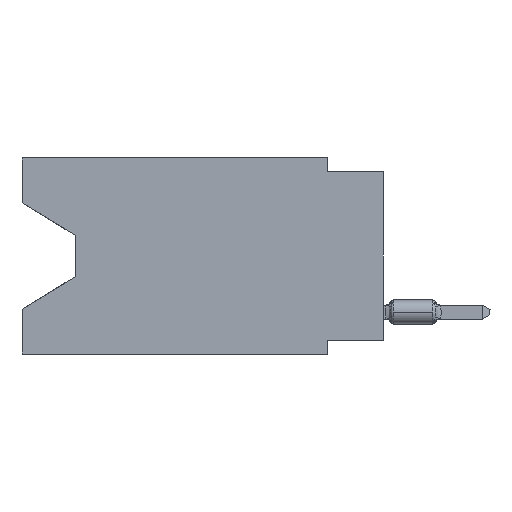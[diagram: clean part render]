
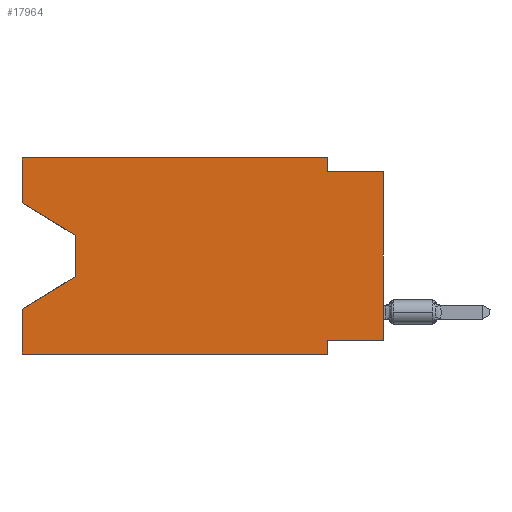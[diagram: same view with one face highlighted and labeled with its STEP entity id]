
A CAD part, left-side view. The second image highlights one B-rep face of the part: STEP entity #17964.
In plain terms, the highlighted planar face has unit normal (-1, 0, 0).
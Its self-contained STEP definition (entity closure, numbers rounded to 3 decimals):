
#676 = CARTESIAN_POINT ( 'NONE',  ( 0., 2.54, -0.635 ) ) ;
#875 = DIRECTION ( 'NONE',  ( 0., 0., -1. ) ) ;
#980 = VECTOR ( 'NONE', #48098, 1000. ) ;
#1937 = VECTOR ( 'NONE', #20062, 1000. ) ;
#3966 = VECTOR ( 'NONE', #53727, 1000. ) ;
#4499 = EDGE_CURVE ( 'NONE', #33399, #41861, #5363, .T. ) ;
#4623 = LINE ( 'NONE', #45652, #40477 ) ;
#4881 = CARTESIAN_POINT ( 'NONE',  ( 0., 2.54, -8.89 ) ) ;
#5284 = CARTESIAN_POINT ( 'NONE',  ( 0., 0., -8.255 ) ) ;
#5363 = LINE ( 'NONE', #25217, #5516 ) ;
#5516 = VECTOR ( 'NONE', #49638, 1000. ) ;
#5627 = AXIS2_PLACEMENT_3D ( 'NONE', #17727, #50053, #875 ) ;
#6495 = ORIENTED_EDGE ( 'NONE', *, *, #13735, .F. ) ;
#6809 = DIRECTION ( 'NONE',  ( 0., -1., 0. ) ) ;
#7273 = CARTESIAN_POINT ( 'NONE',  ( 0., 13.97, -5.385 ) ) ;
#8082 = LINE ( 'NONE', #28492, #21267 ) ;
#8533 = VERTEX_POINT ( 'NONE', #39669 ) ;
#8679 = LINE ( 'NONE', #4881, #52269 ) ;
#10050 = VERTEX_POINT ( 'NONE', #676 ) ;
#10669 = ORIENTED_EDGE ( 'NONE', *, *, #30252, .F. ) ;
#11470 = VECTOR ( 'NONE', #51185, 1000. ) ;
#11529 = VERTEX_POINT ( 'NONE', #7273 ) ;
#11612 = VERTEX_POINT ( 'NONE', #30562 ) ;
#12620 = VECTOR ( 'NONE', #21866, 1000. ) ;
#13368 = PLANE ( 'NONE',  #5627 ) ;
#13735 = EDGE_CURVE ( 'NONE', #29307, #45495, #52917, .T. ) ;
#14941 = LINE ( 'NONE', #31545, #980 ) ;
#15012 = LINE ( 'NONE', #20177, #34600 ) ;
#16884 = CARTESIAN_POINT ( 'NONE',  ( 0., 16.383, 0. ) ) ;
#17579 = ORIENTED_EDGE ( 'NONE', *, *, #43287, .T. ) ;
#17727 = CARTESIAN_POINT ( 'NONE',  ( 0., 16.383, 0. ) ) ;
#17964 = ADVANCED_FACE ( 'NONE', ( #42196 ), #13368, .F. ) ;
#18156 = VECTOR ( 'NONE', #37771, 1000. ) ;
#19597 = EDGE_CURVE ( 'NONE', #11529, #21033, #4623, .T. ) ;
#20062 = DIRECTION ( 'NONE',  ( 0., 0., 1. ) ) ;
#20177 = CARTESIAN_POINT ( 'NONE',  ( 0., 0., -0.635 ) ) ;
#20643 = LINE ( 'NONE', #25277, #18156 ) ;
#21033 = VERTEX_POINT ( 'NONE', #52001 ) ;
#21267 = VECTOR ( 'NONE', #45060, 1000. ) ;
#21480 = DIRECTION ( 'NONE',  ( 0., 0.855, -0.519 ) ) ;
#21866 = DIRECTION ( 'NONE',  ( 0., 0., 1. ) ) ;
#21906 = CARTESIAN_POINT ( 'NONE',  ( 0., 2.54, -8.89 ) ) ;
#24367 = CARTESIAN_POINT ( 'NONE',  ( 0., 13.97, -3.505 ) ) ;
#25217 = CARTESIAN_POINT ( 'NONE',  ( 0., 16.383, -8.89 ) ) ;
#25277 = CARTESIAN_POINT ( 'NONE',  ( 0., 2.54, 0. ) ) ;
#25775 = EDGE_CURVE ( 'NONE', #29307, #40229, #14941, .T. ) ;
#26586 = EDGE_CURVE ( 'NONE', #10050, #11612, #15012, .T. ) ;
#27057 = EDGE_CURVE ( 'NONE', #8533, #10050, #20643, .T. ) ;
#27648 = EDGE_CURVE ( 'NONE', #45495, #8533, #28547, .T. ) ;
#28492 = CARTESIAN_POINT ( 'NONE',  ( 0., 13.97, -3.505 ) ) ;
#28547 = LINE ( 'NONE', #48644, #28632 ) ;
#28632 = VECTOR ( 'NONE', #6809, 1000. ) ;
#29307 = VERTEX_POINT ( 'NONE', #49099 ) ;
#30143 = ORIENTED_EDGE ( 'NONE', *, *, #42589, .T. ) ;
#30252 = EDGE_CURVE ( 'NONE', #50317, #41861, #8679, .T. ) ;
#30560 = LINE ( 'NONE', #38455, #12620 ) ;
#30562 = CARTESIAN_POINT ( 'NONE',  ( 0., 0., -0.635 ) ) ;
#31545 = CARTESIAN_POINT ( 'NONE',  ( 0., 16.383, -2.038 ) ) ;
#33121 = ORIENTED_EDGE ( 'NONE', *, *, #50283, .F. ) ;
#33399 = VERTEX_POINT ( 'NONE', #51357 ) ;
#33839 = CARTESIAN_POINT ( 'NONE',  ( 0., 2.54, -8.255 ) ) ;
#34078 = ORIENTED_EDGE ( 'NONE', *, *, #27057, .F. ) ;
#34600 = VECTOR ( 'NONE', #36224, 1000. ) ;
#36135 = ORIENTED_EDGE ( 'NONE', *, *, #26586, .F. ) ;
#36224 = DIRECTION ( 'NONE',  ( 0., -1., 0. ) ) ;
#37077 = ORIENTED_EDGE ( 'NONE', *, *, #25775, .T. ) ;
#37194 = LINE ( 'NONE', #45340, #3966 ) ;
#37394 = VERTEX_POINT ( 'NONE', #42580 ) ;
#37771 = DIRECTION ( 'NONE',  ( 0., 0., -1. ) ) ;
#38455 = CARTESIAN_POINT ( 'NONE',  ( 0., 16.383, 0. ) ) ;
#38637 = ORIENTED_EDGE ( 'NONE', *, *, #27648, .F. ) ;
#38867 = DIRECTION ( 'NONE',  ( 0., 0., -1. ) ) ;
#39669 = CARTESIAN_POINT ( 'NONE',  ( 0., 2.54, 0. ) ) ;
#40229 = VERTEX_POINT ( 'NONE', #24367 ) ;
#40477 = VECTOR ( 'NONE', #21480, 1000. ) ;
#41279 = ORIENTED_EDGE ( 'NONE', *, *, #4499, .T. ) ;
#41861 = VERTEX_POINT ( 'NONE', #21906 ) ;
#42196 = FACE_OUTER_BOUND ( 'NONE', #42490, .T. ) ;
#42490 = EDGE_LOOP ( 'NONE', ( #37077, #17579, #51332, #33121, #41279, #10669, #43118, #30143, #36135, #34078, #38637, #6495 ) ) ;
#42580 = CARTESIAN_POINT ( 'NONE',  ( 0., 0., -8.255 ) ) ;
#42589 = EDGE_CURVE ( 'NONE', #37394, #11612, #37194, .T. ) ;
#42793 = LINE ( 'NONE', #5284, #11470 ) ;
#43118 = ORIENTED_EDGE ( 'NONE', *, *, #45242, .F. ) ;
#43287 = EDGE_CURVE ( 'NONE', #40229, #11529, #8082, .T. ) ;
#45060 = DIRECTION ( 'NONE',  ( 0., 0., -1. ) ) ;
#45242 = EDGE_CURVE ( 'NONE', #37394, #50317, #42793, .T. ) ;
#45340 = CARTESIAN_POINT ( 'NONE',  ( 0., 0., 0. ) ) ;
#45495 = VERTEX_POINT ( 'NONE', #16884 ) ;
#45652 = CARTESIAN_POINT ( 'NONE',  ( 0., 13.97, -5.385 ) ) ;
#48098 = DIRECTION ( 'NONE',  ( 0., -0.855, -0.519 ) ) ;
#48644 = CARTESIAN_POINT ( 'NONE',  ( 0., 16.383, 0. ) ) ;
#48849 = CARTESIAN_POINT ( 'NONE',  ( 0., 16.383, 0. ) ) ;
#49099 = CARTESIAN_POINT ( 'NONE',  ( 0., 16.383, -2.038 ) ) ;
#49638 = DIRECTION ( 'NONE',  ( 0., -1., 0. ) ) ;
#50053 = DIRECTION ( 'NONE',  ( 1., 0., 0. ) ) ;
#50283 = EDGE_CURVE ( 'NONE', #33399, #21033, #30560, .T. ) ;
#50317 = VERTEX_POINT ( 'NONE', #33839 ) ;
#51185 = DIRECTION ( 'NONE',  ( 0., 1., 0. ) ) ;
#51332 = ORIENTED_EDGE ( 'NONE', *, *, #19597, .T. ) ;
#51357 = CARTESIAN_POINT ( 'NONE',  ( 0., 16.383, -8.89 ) ) ;
#52001 = CARTESIAN_POINT ( 'NONE',  ( 0., 16.383, -6.852 ) ) ;
#52269 = VECTOR ( 'NONE', #38867, 1000. ) ;
#52917 = LINE ( 'NONE', #48849, #1937 ) ;
#53727 = DIRECTION ( 'NONE',  ( 0., 0., 1. ) ) ;
